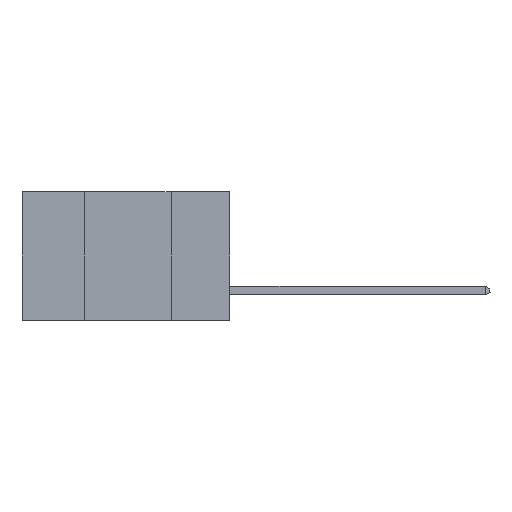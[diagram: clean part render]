
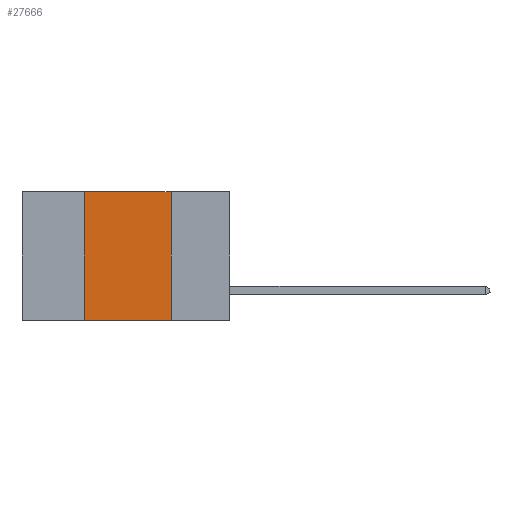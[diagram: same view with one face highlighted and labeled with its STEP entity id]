
A CAD part, left-side view. The second image highlights one B-rep face of the part: STEP entity #27666.
In plain terms, the highlighted planar face has unit normal (-1, 0, 0).
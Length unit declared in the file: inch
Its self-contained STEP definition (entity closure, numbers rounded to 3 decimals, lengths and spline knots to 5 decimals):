
#431 = LINE ( 'NONE', #5211, #27484 ) ;
#449 = EDGE_CURVE ( 'NONE', #4347, #21558, #2563, .T. ) ;
#2116 = ORIENTED_EDGE ( 'NONE', *, *, #449, .F. ) ;
#2563 = LINE ( 'NONE', #22193, #4073 ) ;
#4073 = VECTOR ( 'NONE', #26475, 39.37008 ) ;
#4214 = DIRECTION ( 'NONE',  ( 1., 0., 0. ) ) ;
#4347 = VERTEX_POINT ( 'NONE', #27276 ) ;
#5211 = CARTESIAN_POINT ( 'NONE',  ( 0., 0.17, 0. ) ) ;
#6185 = DIRECTION ( 'NONE',  ( 0., 0., -1. ) ) ;
#7493 = EDGE_CURVE ( 'NONE', #21558, #11982, #22412, .T. ) ;
#7600 = LINE ( 'NONE', #14592, #20952 ) ;
#10258 = DIRECTION ( 'NONE',  ( 0., -1., 0. ) ) ;
#10420 = CARTESIAN_POINT ( 'NONE',  ( 0., 0.17, -0.37 ) ) ;
#11827 = EDGE_LOOP ( 'NONE', ( #16900, #16236, #2116, #18975 ) ) ;
#11982 = VERTEX_POINT ( 'NONE', #19875 ) ;
#14144 = CARTESIAN_POINT ( 'NONE',  ( 0., 0.6, 0. ) ) ;
#14592 = CARTESIAN_POINT ( 'NONE',  ( 0., 0.6, -0.37 ) ) ;
#16236 = ORIENTED_EDGE ( 'NONE', *, *, #7493, .F. ) ;
#16267 = DIRECTION ( 'NONE',  ( 0., -1., 0. ) ) ;
#16694 = DIRECTION ( 'NONE',  ( 0., 0., -1. ) ) ;
#16900 = ORIENTED_EDGE ( 'NONE', *, *, #26683, .F. ) ;
#18372 = EDGE_CURVE ( 'NONE', #4347, #21084, #7600, .T. ) ;
#18975 = ORIENTED_EDGE ( 'NONE', *, *, #18372, .T. ) ;
#19875 = CARTESIAN_POINT ( 'NONE',  ( 0., 0.17, 0. ) ) ;
#19979 = PLANE ( 'NONE',  #24403 ) ;
#20278 = CARTESIAN_POINT ( 'NONE',  ( 0., 0.6, 0. ) ) ;
#20952 = VECTOR ( 'NONE', #10258, 39.37008 ) ;
#21084 = VERTEX_POINT ( 'NONE', #10420 ) ;
#21558 = VERTEX_POINT ( 'NONE', #26474 ) ;
#22193 = CARTESIAN_POINT ( 'NONE',  ( 0., 0.42, 0. ) ) ;
#22412 = LINE ( 'NONE', #14144, #29592 ) ;
#24403 = AXIS2_PLACEMENT_3D ( 'NONE', #20278, #4214, #6185 ) ;
#26474 = CARTESIAN_POINT ( 'NONE',  ( 0., 0.42, 0. ) ) ;
#26475 = DIRECTION ( 'NONE',  ( 0., 0., 1. ) ) ;
#26683 = EDGE_CURVE ( 'NONE', #11982, #21084, #431, .T. ) ;
#27276 = CARTESIAN_POINT ( 'NONE',  ( 0., 0.42, -0.37 ) ) ;
#27484 = VECTOR ( 'NONE', #16694, 39.37008 ) ;
#27666 = ADVANCED_FACE ( 'NONE', ( #28522 ), #19979, .F. ) ;
#28522 = FACE_OUTER_BOUND ( 'NONE', #11827, .T. ) ;
#29592 = VECTOR ( 'NONE', #16267, 39.37008 ) ;
